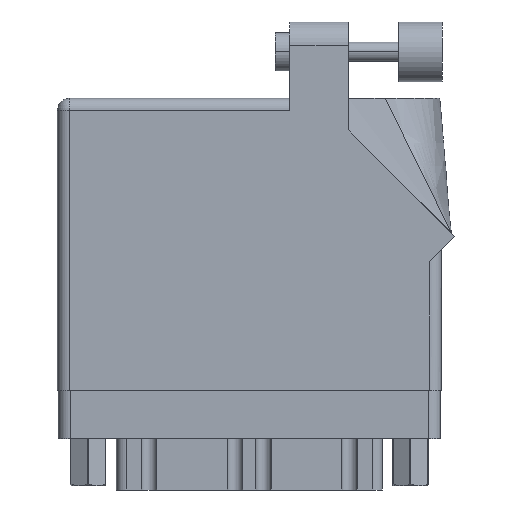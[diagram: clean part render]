
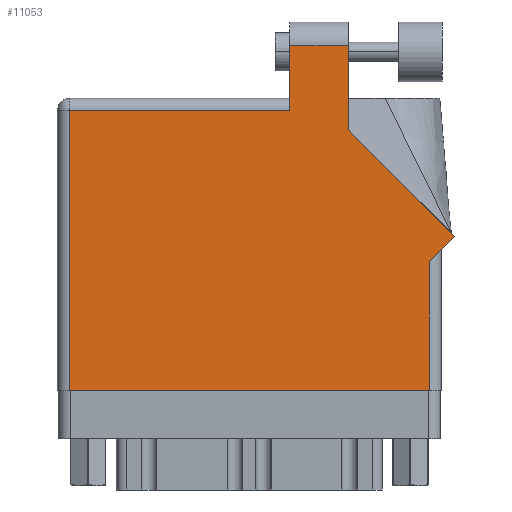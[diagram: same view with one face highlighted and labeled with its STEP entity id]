
A CAD part, front view. The second image highlights one B-rep face of the part: STEP entity #11053.
In plain terms, the highlighted face is planar.
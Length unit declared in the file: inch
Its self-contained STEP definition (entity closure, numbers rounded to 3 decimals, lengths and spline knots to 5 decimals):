
#1179 = DIRECTION ( 'NONE',  ( 0., 0., -1. ) ) ;
#1926 = CARTESIAN_POINT ( 'NONE',  ( 1.948, 0.737, 0. ) ) ;
#2622 = ORIENTED_EDGE ( 'NONE', *, *, #38110, .T. ) ;
#3413 = CARTESIAN_POINT ( 'NONE',  ( 1.217, 1.468, 0. ) ) ;
#4000 = VECTOR ( 'NONE', #31091, 39.37008 ) ;
#4258 = CARTESIAN_POINT ( 'NONE',  ( 1.524, 1.805, 0. ) ) ;
#5088 = CARTESIAN_POINT ( 'NONE',  ( 1.524, 1.36442, 0. ) ) ;
#5491 = DIRECTION ( 'NONE',  ( -1., 0., 0. ) ) ;
#5646 = LINE ( 'NONE', #34915, #16082 ) ;
#5688 = CARTESIAN_POINT ( 'NONE',  ( 0.062, 0., 0. ) ) ;
#5722 = CARTESIAN_POINT ( 'NONE',  ( 0., 1.53, 0. ) ) ;
#6295 = CARTESIAN_POINT ( 'NONE',  ( 0., 0., 0. ) ) ;
#8013 = VERTEX_POINT ( 'NONE', #4258 ) ;
#8214 = VERTEX_POINT ( 'NONE', #31154 ) ;
#8746 = EDGE_CURVE ( 'NONE', #8214, #27441, #38026, .T. ) ;
#8765 = VECTOR ( 'NONE', #15092, 39.37008 ) ;
#9254 = EDGE_CURVE ( 'NONE', #36244, #32642, #19954, .T. ) ;
#10814 = VECTOR ( 'NONE', #13009, 39.37008 ) ;
#11053 = ADVANCED_FACE ( 'NONE', ( #38109 ), #34758, .F. ) ;
#11490 = LINE ( 'NONE', #40515, #8765 ) ;
#12174 = VECTOR ( 'NONE', #20946, 39.37008 ) ;
#12324 = LINE ( 'NONE', #26969, #41813 ) ;
#12794 = LINE ( 'NONE', #16399, #16497 ) ;
#13009 = DIRECTION ( 'NONE',  ( 0., -1., 0. ) ) ;
#13886 = VERTEX_POINT ( 'NONE', #3413 ) ;
#15092 = DIRECTION ( 'NONE',  ( 0.707, 0.707, 0. ) ) ;
#16082 = VECTOR ( 'NONE', #19355, 39.37008 ) ;
#16399 = CARTESIAN_POINT ( 'NONE',  ( 1.524, 1.36442, 0. ) ) ;
#16497 = VECTOR ( 'NONE', #27431, 39.37008 ) ;
#16624 = CARTESIAN_POINT ( 'NONE',  ( 1.217, 1.53, 0. ) ) ;
#19355 = DIRECTION ( 'NONE',  ( 0., -1., 0. ) ) ;
#19828 = DIRECTION ( 'NONE',  ( -0.707, 0.707, 0. ) ) ;
#19954 = LINE ( 'NONE', #1926, #24688 ) ;
#20153 = EDGE_CURVE ( 'NONE', #32642, #8214, #11490, .T. ) ;
#20946 = DIRECTION ( 'NONE',  ( 1., 0., 0. ) ) ;
#22439 = ORIENTED_EDGE ( 'NONE', *, *, #9254, .T. ) ;
#23570 = LINE ( 'NONE', #16624, #10814 ) ;
#23759 = CARTESIAN_POINT ( 'NONE',  ( 1.217, 1.805, 0. ) ) ;
#23855 = ORIENTED_EDGE ( 'NONE', *, *, #31778, .T. ) ;
#24537 = LINE ( 'NONE', #6295, #12174 ) ;
#24688 = VECTOR ( 'NONE', #30265, 39.37008 ) ;
#25841 = CARTESIAN_POINT ( 'NONE',  ( 1.217, 1.805, 0. ) ) ;
#26209 = EDGE_LOOP ( 'NONE', ( #33355, #46630, #23855, #2622, #30061, #40931, #22439, #38464, #26375 ) ) ;
#26375 = ORIENTED_EDGE ( 'NONE', *, *, #8746, .T. ) ;
#26969 = CARTESIAN_POINT ( 'NONE',  ( 0., 1.468, 0. ) ) ;
#27431 = DIRECTION ( 'NONE',  ( 0., 1., 0. ) ) ;
#27441 = VERTEX_POINT ( 'NONE', #5088 ) ;
#27660 = EDGE_CURVE ( 'NONE', #41545, #36244, #24537, .T. ) ;
#29207 = LINE ( 'NONE', #25841, #4000 ) ;
#29898 = CARTESIAN_POINT ( 'NONE',  ( 1.948, 0., 0. ) ) ;
#30061 = ORIENTED_EDGE ( 'NONE', *, *, #45034, .T. ) ;
#30265 = DIRECTION ( 'NONE',  ( 0., 1., 0. ) ) ;
#31091 = DIRECTION ( 'NONE',  ( -1., 0., 0. ) ) ;
#31154 = CARTESIAN_POINT ( 'NONE',  ( 2.08071, 0.80771, 0. ) ) ;
#31778 = EDGE_CURVE ( 'NONE', #32224, #13886, #23570, .T. ) ;
#32224 = VERTEX_POINT ( 'NONE', #23759 ) ;
#32591 = VERTEX_POINT ( 'NONE', #43628 ) ;
#32642 = VERTEX_POINT ( 'NONE', #37108 ) ;
#33035 = VECTOR ( 'NONE', #19828, 39.37008 ) ;
#33355 = ORIENTED_EDGE ( 'NONE', *, *, #37937, .T. ) ;
#34381 = EDGE_CURVE ( 'NONE', #8013, #32224, #29207, .T. ) ;
#34758 = PLANE ( 'NONE',  #37225 ) ;
#34915 = CARTESIAN_POINT ( 'NONE',  ( 0.062, 0., 0. ) ) ;
#36244 = VERTEX_POINT ( 'NONE', #29898 ) ;
#37108 = CARTESIAN_POINT ( 'NONE',  ( 1.948, 0.675, 0. ) ) ;
#37225 = AXIS2_PLACEMENT_3D ( 'NONE', #5722, #1179, #5491 ) ;
#37937 = EDGE_CURVE ( 'NONE', #27441, #8013, #12794, .T. ) ;
#38026 = LINE ( 'NONE', #42342, #33035 ) ;
#38110 = EDGE_CURVE ( 'NONE', #13886, #32591, #12324, .T. ) ;
#38109 = FACE_OUTER_BOUND ( 'NONE', #26209, .T. ) ;
#38464 = ORIENTED_EDGE ( 'NONE', *, *, #20153, .T. ) ;
#39150 = DIRECTION ( 'NONE',  ( -1., 0., 0. ) ) ;
#40515 = CARTESIAN_POINT ( 'NONE',  ( 2.01, 0.737, 0. ) ) ;
#40931 = ORIENTED_EDGE ( 'NONE', *, *, #27660, .T. ) ;
#41545 = VERTEX_POINT ( 'NONE', #5688 ) ;
#41813 = VECTOR ( 'NONE', #39150, 39.37008 ) ;
#42342 = CARTESIAN_POINT ( 'NONE',  ( 2.08071, 0.80771, 0. ) ) ;
#43628 = CARTESIAN_POINT ( 'NONE',  ( 0.062, 1.468, 0. ) ) ;
#45034 = EDGE_CURVE ( 'NONE', #32591, #41545, #5646, .T. ) ;
#46630 = ORIENTED_EDGE ( 'NONE', *, *, #34381, .T. ) ;
